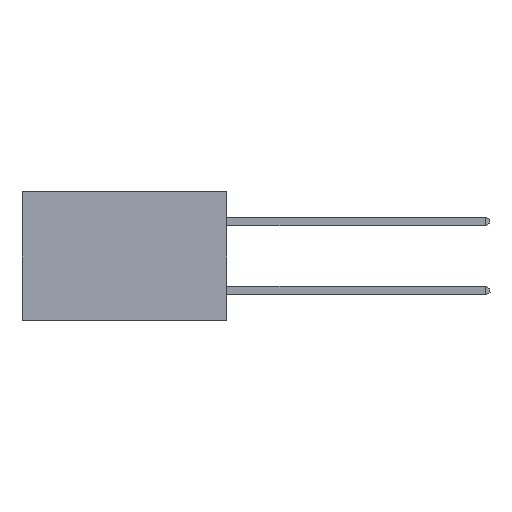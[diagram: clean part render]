
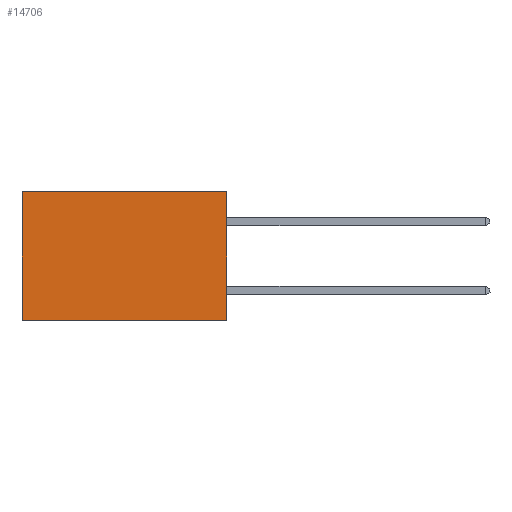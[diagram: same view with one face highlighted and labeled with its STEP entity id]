
A CAD part, left-side view. The second image highlights one B-rep face of the part: STEP entity #14706.
In plain terms, the highlighted planar face has unit normal (-1, 0, 0).
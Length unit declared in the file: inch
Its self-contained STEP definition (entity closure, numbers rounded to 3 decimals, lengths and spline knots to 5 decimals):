
#838 = CARTESIAN_POINT ( 'NONE',  ( 0.277, 0., 0. ) ) ;
#1277 = DIRECTION ( 'NONE',  ( 0., 0., -1. ) ) ;
#1337 = ORIENTED_EDGE ( 'NONE', *, *, #3866, .F. ) ;
#1372 = LINE ( 'NONE', #22673, #13027 ) ;
#3013 = FACE_OUTER_BOUND ( 'NONE', #30377, .T. ) ;
#3367 = DIRECTION ( 'NONE',  ( 0., 1., 0. ) ) ;
#3866 = EDGE_CURVE ( 'NONE', #10329, #21749, #1372, .T. ) ;
#4774 = EDGE_CURVE ( 'NONE', #27039, #21749, #6385, .T. ) ;
#5643 = CARTESIAN_POINT ( 'NONE',  ( 0.277, 0., -0.37 ) ) ;
#6385 = LINE ( 'NONE', #27852, #31935 ) ;
#6588 = ORIENTED_EDGE ( 'NONE', *, *, #12930, .F. ) ;
#6665 = VECTOR ( 'NONE', #3367, 39.37008 ) ;
#7026 = DIRECTION ( 'NONE',  ( 0., 0., -1. ) ) ;
#10329 = VERTEX_POINT ( 'NONE', #5643 ) ;
#11184 = PLANE ( 'NONE',  #12400 ) ;
#12400 = AXIS2_PLACEMENT_3D ( 'NONE', #13577, #16157, #1277 ) ;
#12557 = EDGE_CURVE ( 'NONE', #23393, #27039, #13246, .T. ) ;
#12930 = EDGE_CURVE ( 'NONE', #23393, #10329, #16329, .T. ) ;
#13027 = VECTOR ( 'NONE', #21971, 39.37008 ) ;
#13246 = LINE ( 'NONE', #838, #6665 ) ;
#13577 = CARTESIAN_POINT ( 'NONE',  ( 0.277, 0., -0.37 ) ) ;
#14706 = ADVANCED_FACE ( 'NONE', ( #3013 ), #11184, .F. ) ;
#16157 = DIRECTION ( 'NONE',  ( 1., 0., 0. ) ) ;
#16329 = LINE ( 'NONE', #19404, #22166 ) ;
#17226 = ORIENTED_EDGE ( 'NONE', *, *, #12557, .T. ) ;
#17860 = CARTESIAN_POINT ( 'NONE',  ( 0.277, 0., 0. ) ) ;
#19259 = CARTESIAN_POINT ( 'NONE',  ( 0.277, 0.59, -0.37 ) ) ;
#19404 = CARTESIAN_POINT ( 'NONE',  ( 0.277, 0., -0.37 ) ) ;
#21341 = ORIENTED_EDGE ( 'NONE', *, *, #4774, .T. ) ;
#21749 = VERTEX_POINT ( 'NONE', #19259 ) ;
#21971 = DIRECTION ( 'NONE',  ( 0., 1., 0. ) ) ;
#22166 = VECTOR ( 'NONE', #7026, 39.37008 ) ;
#22673 = CARTESIAN_POINT ( 'NONE',  ( 0.277, 0., -0.37 ) ) ;
#23393 = VERTEX_POINT ( 'NONE', #17860 ) ;
#27039 = VERTEX_POINT ( 'NONE', #29850 ) ;
#27701 = DIRECTION ( 'NONE',  ( 0., 0., -1. ) ) ;
#27852 = CARTESIAN_POINT ( 'NONE',  ( 0.277, 0.59, -0.37 ) ) ;
#29850 = CARTESIAN_POINT ( 'NONE',  ( 0.277, 0.59, 0. ) ) ;
#30377 = EDGE_LOOP ( 'NONE', ( #21341, #1337, #6588, #17226 ) ) ;
#31935 = VECTOR ( 'NONE', #27701, 39.37008 ) ;
